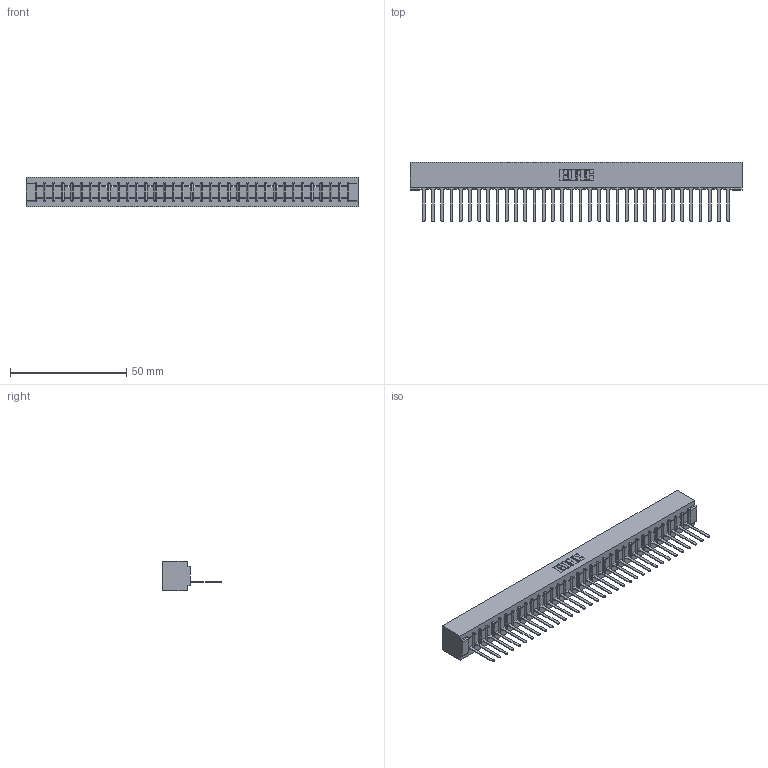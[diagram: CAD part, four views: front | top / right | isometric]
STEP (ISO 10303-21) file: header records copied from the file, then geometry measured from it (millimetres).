
FILE_DESCRIPTION (( 'STEP AP203' ), '1' );
FILE_NAME ('357-034-447-101.STEP', '2020-10-02T09:44:25', ( '' ), ( '' ), 'SwSTEP 2.0', 'SolidWorks 2020', '' );
FILE_SCHEMA (( 'CONFIG_CONTROL_DESIGN' ));
Length unit declared in the file: inch
Products named in the file (3): 307-290-001_547; 357-034-447-101; 307 Part_No Mounting Lugs
Assembly tree (35 placements, depth 2):
  357-034-447-101
    307 Part_No Mounting Lugs
    307-290-001_547  x34
Bounding box: 142.6 x 25.43 x 12.7 mm (x, y, z)
Volume: 15345.4 mm3; surface area: 16791.2 mm2
Topology: 35 solids, 35 shells, 2049 faces, 5807 edges, 3730 vertices
Faces by surface type: plane 1324, cylinder 655, sphere 70
Entity records: 29824 total; most frequent: CARTESIAN_POINT 5020, ORIENTED_EDGE 5006, DIRECTION 4885, EDGE_CURVE 2503, LINE 1919, VECTOR 1919, VERTEX_POINT 1618, AXIS2_PLACEMENT_3D 1483
